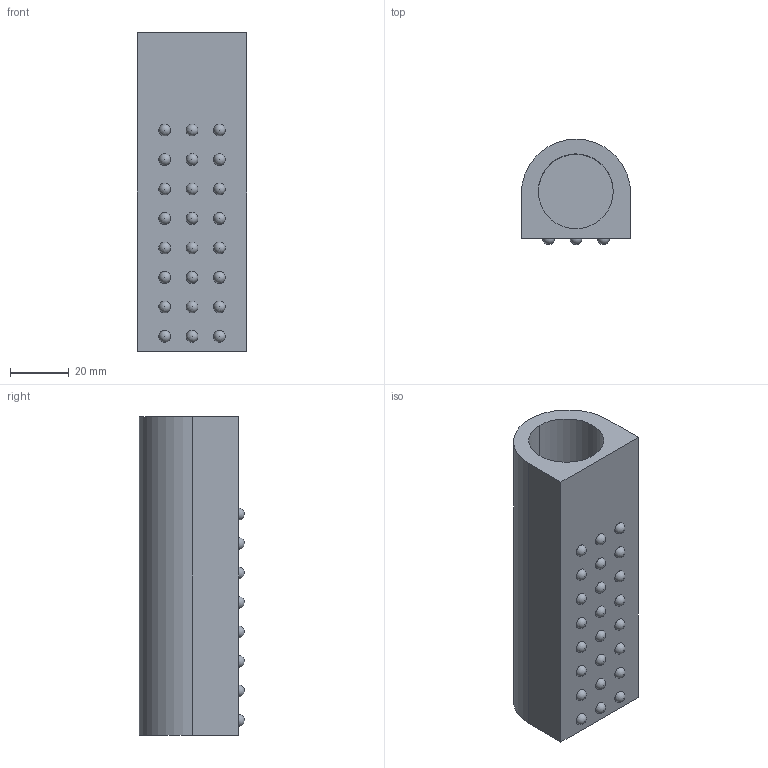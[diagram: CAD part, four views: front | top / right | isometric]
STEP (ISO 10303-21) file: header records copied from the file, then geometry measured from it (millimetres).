
FILE_DESCRIPTION (( 'STEP AP214' ), '1' );
FILE_NAME ('Buffer_Tube_2a.STEP', '2013-09-01T16:38:16', ( 'Asher' ), ( '' ), 'SwSTEP 2.0', 'SolidWorks 2013', '' );
FILE_SCHEMA (( 'AUTOMOTIVE_DESIGN' ));
Length unit declared in the file: millimetre
Products named in the file (1): Buffer_Tube_2a
Bounding box: 37.13 x 35.66 x 108 mm (x, y, z)
Volume: 74584.9 mm3; surface area: 23137.5 mm2
Topology: 1 solids, 1 shells, 33 faces, 138 edges, 108 vertices
Faces by surface type: sphere 24, plane 6, cylinder 3
Entity records: 992 total; most frequent: DIRECTION 188, CARTESIAN_POINT 160, ORIENTED_EDGE 132, AXIS2_PLACEMENT_3D 88, EDGE_CURVE 66, VERTEX_POINT 60, EDGE_LOOP 58, CIRCLE 54
